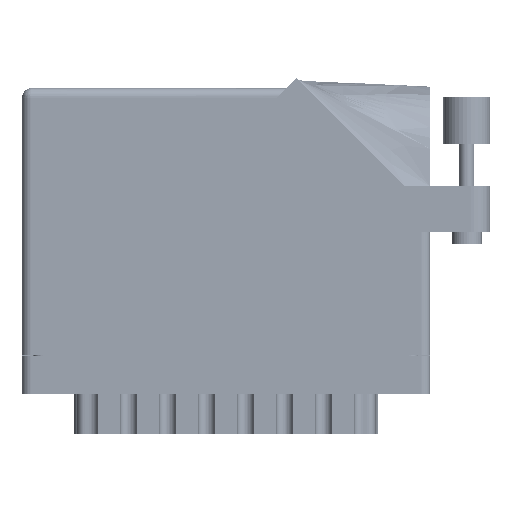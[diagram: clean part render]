
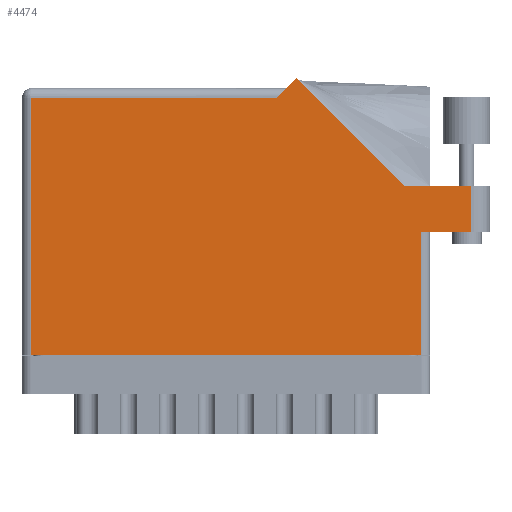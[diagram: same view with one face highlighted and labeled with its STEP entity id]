
A CAD part, front view. The second image highlights one B-rep face of the part: STEP entity #4474.
In plain terms, the highlighted face is planar.
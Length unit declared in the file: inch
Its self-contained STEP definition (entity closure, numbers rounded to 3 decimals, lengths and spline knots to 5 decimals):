
#9 = CARTESIAN_POINT ( 'NONE',  ( 2.55242, 1.122, 0. ) ) ;
#509 = ORIENTED_EDGE ( 'NONE', *, *, #38835, .T. ) ;
#3171 = LINE ( 'NONE', #24978, #53023 ) ;
#3480 = DIRECTION ( 'NONE',  ( 0., 0., -1. ) ) ;
#4474 = ADVANCED_FACE ( 'NONE', ( #71441 ), #26734, .F. ) ;
#4641 = VERTEX_POINT ( 'NONE', #16730 ) ;
#8147 = ORIENTED_EDGE ( 'NONE', *, *, #59073, .T. ) ;
#8493 = ORIENTED_EDGE ( 'NONE', *, *, #12309, .T. ) ;
#8555 = AXIS2_PLACEMENT_3D ( 'NONE', #21197, #3480, #72153 ) ;
#9220 = EDGE_CURVE ( 'NONE', #62730, #61756, #32572, .T. ) ;
#9986 = VECTOR ( 'NONE', #35137, 39.37008 ) ;
#11636 = CARTESIAN_POINT ( 'NONE',  ( 1.758, 1.775, 0. ) ) ;
#12309 = EDGE_CURVE ( 'NONE', #4641, #16928, #38660, .T. ) ;
#14910 = VECTOR ( 'NONE', #44736, 39.37008 ) ;
#15071 = LINE ( 'NONE', #53521, #18341 ) ;
#16730 = CARTESIAN_POINT ( 'NONE',  ( 2.993, 0.815, 0. ) ) ;
#16928 = VERTEX_POINT ( 'NONE', #64960 ) ;
#17357 = LINE ( 'NONE', #50617, #14910 ) ;
#17600 = EDGE_CURVE ( 'NONE', #29351, #50205, #39730, .T. ) ;
#17662 = CARTESIAN_POINT ( 'NONE',  ( 2.656, 0.815, 0. ) ) ;
#18341 = VECTOR ( 'NONE', #66042, 39.37008 ) ;
#18770 = ORIENTED_EDGE ( 'NONE', *, *, #44826, .T. ) ;
#19944 = EDGE_CURVE ( 'NONE', #21631, #29351, #39555, .T. ) ;
#21197 = CARTESIAN_POINT ( 'NONE',  ( 0., 1.775, 0. ) ) ;
#21631 = VERTEX_POINT ( 'NONE', #25020 ) ;
#24978 = CARTESIAN_POINT ( 'NONE',  ( 3.118, 1.122, 0. ) ) ;
#25020 = CARTESIAN_POINT ( 'NONE',  ( 2.55242, 1.122, 0. ) ) ;
#25126 = VERTEX_POINT ( 'NONE', #43998 ) ;
#26564 = VERTEX_POINT ( 'NONE', #60455 ) ;
#26734 = PLANE ( 'NONE',  #8555 ) ;
#26930 = LINE ( 'NONE', #67182, #9986 ) ;
#27351 = CARTESIAN_POINT ( 'NONE',  ( 2.656, 0.815, 0. ) ) ;
#29351 = VERTEX_POINT ( 'NONE', #35368 ) ;
#29799 = DIRECTION ( 'NONE',  ( 1., 0., 0. ) ) ;
#30942 = VECTOR ( 'NONE', #61173, 39.37008 ) ;
#32572 = LINE ( 'NONE', #27351, #47120 ) ;
#32759 = CARTESIAN_POINT ( 'NONE',  ( 2.993, 1.122, 0. ) ) ;
#34028 = VECTOR ( 'NONE', #29799, 39.37008 ) ;
#35137 = DIRECTION ( 'NONE',  ( 0., -1., 0. ) ) ;
#35368 = CARTESIAN_POINT ( 'NONE',  ( 1.82871, 1.84571, 0. ) ) ;
#38473 = DIRECTION ( 'NONE',  ( 0., 1., 0. ) ) ;
#38660 = LINE ( 'NONE', #32759, #30942 ) ;
#38835 = EDGE_CURVE ( 'NONE', #25126, #26564, #26930, .T. ) ;
#39555 = LINE ( 'NONE', #9, #41336 ) ;
#39730 = LINE ( 'NONE', #11636, #45367 ) ;
#40906 = LINE ( 'NONE', #69314, #34028 ) ;
#41336 = VECTOR ( 'NONE', #62070, 39.37008 ) ;
#43998 = CARTESIAN_POINT ( 'NONE',  ( 0.062, 1.713, 0. ) ) ;
#44736 = DIRECTION ( 'NONE',  ( -1., 0., 0. ) ) ;
#44826 = EDGE_CURVE ( 'NONE', #16928, #21631, #3171, .T. ) ;
#45301 = ORIENTED_EDGE ( 'NONE', *, *, #17600, .T. ) ;
#45367 = VECTOR ( 'NONE', #56703, 39.37008 ) ;
#47044 = EDGE_LOOP ( 'NONE', ( #66754, #8493, #18770, #49165, #45301, #63587, #509, #8147, #49630 ) ) ;
#47120 = VECTOR ( 'NONE', #38473, 39.37008 ) ;
#49165 = ORIENTED_EDGE ( 'NONE', *, *, #19944, .T. ) ;
#49630 = ORIENTED_EDGE ( 'NONE', *, *, #9220, .T. ) ;
#50205 = VERTEX_POINT ( 'NONE', #64421 ) ;
#50617 = CARTESIAN_POINT ( 'NONE',  ( 0., 1.713, 0. ) ) ;
#53023 = VECTOR ( 'NONE', #70409, 39.37008 ) ;
#53521 = CARTESIAN_POINT ( 'NONE',  ( 0., 0., 0. ) ) ;
#54715 = EDGE_CURVE ( 'NONE', #61756, #4641, #40906, .T. ) ;
#56703 = DIRECTION ( 'NONE',  ( -0.707, -0.707, 0. ) ) ;
#59073 = EDGE_CURVE ( 'NONE', #26564, #62730, #15071, .T. ) ;
#59568 = CARTESIAN_POINT ( 'NONE',  ( 2.656, 0., 0. ) ) ;
#60126 = EDGE_CURVE ( 'NONE', #50205, #25126, #17357, .T. ) ;
#60455 = CARTESIAN_POINT ( 'NONE',  ( 0.062, 0., 0. ) ) ;
#61173 = DIRECTION ( 'NONE',  ( 0., 1., 0. ) ) ;
#61756 = VERTEX_POINT ( 'NONE', #17662 ) ;
#62070 = DIRECTION ( 'NONE',  ( -0.707, 0.707, 0. ) ) ;
#62730 = VERTEX_POINT ( 'NONE', #59568 ) ;
#63587 = ORIENTED_EDGE ( 'NONE', *, *, #60126, .T. ) ;
#64421 = CARTESIAN_POINT ( 'NONE',  ( 1.696, 1.713, 0. ) ) ;
#64960 = CARTESIAN_POINT ( 'NONE',  ( 2.993, 1.122, 0. ) ) ;
#66042 = DIRECTION ( 'NONE',  ( 1., 0., 0. ) ) ;
#66754 = ORIENTED_EDGE ( 'NONE', *, *, #54715, .T. ) ;
#67182 = CARTESIAN_POINT ( 'NONE',  ( 0.062, 0., 0. ) ) ;
#69314 = CARTESIAN_POINT ( 'NONE',  ( 2.718, 0.815, 0. ) ) ;
#70409 = DIRECTION ( 'NONE',  ( -1., 0., 0. ) ) ;
#71441 = FACE_OUTER_BOUND ( 'NONE', #47044, .T. ) ;
#72153 = DIRECTION ( 'NONE',  ( -1., 0., 0. ) ) ;
